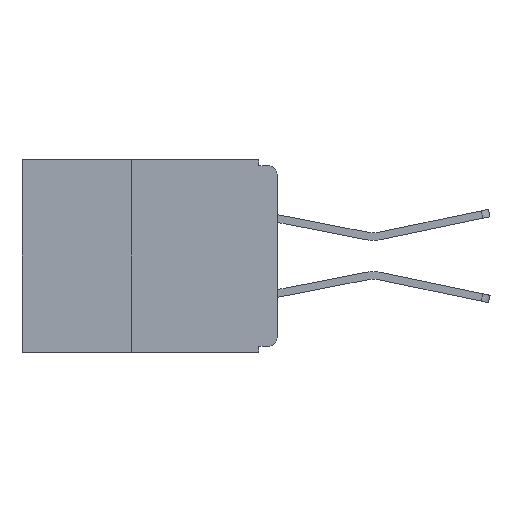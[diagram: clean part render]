
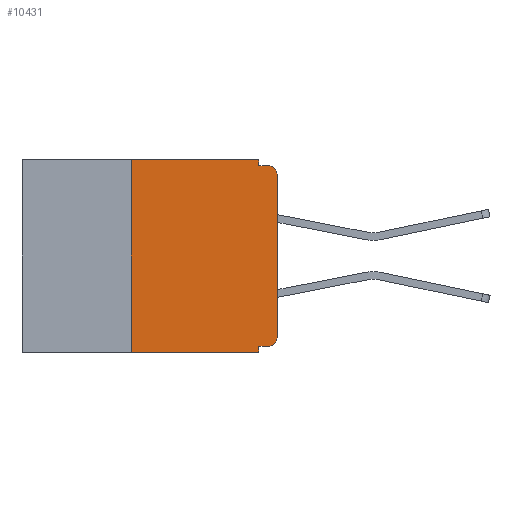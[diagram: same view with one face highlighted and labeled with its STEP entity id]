
A CAD part, left-side view. The second image highlights one B-rep face of the part: STEP entity #10431.
In plain terms, the highlighted planar face has unit normal (-1, 0, 0).
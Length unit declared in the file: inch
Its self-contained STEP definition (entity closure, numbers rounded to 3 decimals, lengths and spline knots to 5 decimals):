
#203 = CARTESIAN_POINT ( 'NONE',  ( 0., 0.031, 0. ) ) ;
#400 = CARTESIAN_POINT ( 'NONE',  ( 0., 0., -0.01 ) ) ;
#616 = ORIENTED_EDGE ( 'NONE', *, *, #10566, .F. ) ;
#731 = EDGE_CURVE ( 'NONE', #3363, #6437, #2843, .T. ) ;
#968 = CARTESIAN_POINT ( 'NONE',  ( 0., 0.015, -0.025 ) ) ;
#974 = LINE ( 'NONE', #12995, #9092 ) ;
#1455 = VERTEX_POINT ( 'NONE', #6132 ) ;
#1554 = VECTOR ( 'NONE', #11753, 39.37008 ) ;
#1560 = CARTESIAN_POINT ( 'NONE',  ( 0., 0.25, 0. ) ) ;
#1798 = ORIENTED_EDGE ( 'NONE', *, *, #11743, .F. ) ;
#1991 = PLANE ( 'NONE',  #2355 ) ;
#2018 = DIRECTION ( 'NONE',  ( 0., 0., -1. ) ) ;
#2137 = LINE ( 'NONE', #8072, #4761 ) ;
#2355 = AXIS2_PLACEMENT_3D ( 'NONE', #3112, #4258, #11383 ) ;
#2638 = AXIS2_PLACEMENT_3D ( 'NONE', #8622, #8341, #4077 ) ;
#2678 = ORIENTED_EDGE ( 'NONE', *, *, #10644, .F. ) ;
#2767 = DIRECTION ( 'NONE',  ( 0., 1., 0. ) ) ;
#2843 = CIRCLE ( 'NONE', #2638, 0.015 ) ;
#3112 = CARTESIAN_POINT ( 'NONE',  ( 0., 0.437, 0. ) ) ;
#3325 = CARTESIAN_POINT ( 'NONE',  ( 0., 0.031, -0.01 ) ) ;
#3348 = VERTEX_POINT ( 'NONE', #3325 ) ;
#3363 = VERTEX_POINT ( 'NONE', #12486 ) ;
#3395 = ORIENTED_EDGE ( 'NONE', *, *, #13267, .F. ) ;
#3677 = DIRECTION ( 'NONE',  ( 0., -1., 0. ) ) ;
#4077 = DIRECTION ( 'NONE',  ( 0., 0., -1. ) ) ;
#4258 = DIRECTION ( 'NONE',  ( 1., 0., 0. ) ) ;
#4278 = ORIENTED_EDGE ( 'NONE', *, *, #731, .T. ) ;
#4408 = DIRECTION ( 'NONE',  ( 0., -1., 0. ) ) ;
#4569 = VECTOR ( 'NONE', #11627, 39.37008 ) ;
#4761 = VECTOR ( 'NONE', #2767, 39.37008 ) ;
#4828 = LINE ( 'NONE', #10770, #1554 ) ;
#4979 = VECTOR ( 'NONE', #5648, 39.37008 ) ;
#5104 = CARTESIAN_POINT ( 'NONE',  ( 0., 0.25, -0.33 ) ) ;
#5451 = ORIENTED_EDGE ( 'NONE', *, *, #7136, .T. ) ;
#5579 = LINE ( 'NONE', #400, #7977 ) ;
#5647 = VECTOR ( 'NONE', #12519, 39.37008 ) ;
#5648 = DIRECTION ( 'NONE',  ( 0., 0., -1. ) ) ;
#5718 = ORIENTED_EDGE ( 'NONE', *, *, #7608, .T. ) ;
#5966 = EDGE_CURVE ( 'NONE', #3363, #12352, #2137, .T. ) ;
#6132 = CARTESIAN_POINT ( 'NONE',  ( 0., 0.015, -0.01 ) ) ;
#6177 = ORIENTED_EDGE ( 'NONE', *, *, #6625, .F. ) ;
#6437 = VERTEX_POINT ( 'NONE', #12530 ) ;
#6625 = EDGE_CURVE ( 'NONE', #3348, #1455, #5579, .T. ) ;
#6684 = VERTEX_POINT ( 'NONE', #11894 ) ;
#6759 = EDGE_CURVE ( 'NONE', #6437, #6684, #974, .T. ) ;
#6869 = EDGE_LOOP ( 'NONE', ( #11303, #5718, #6177, #2678, #1798, #616, #5451, #3395, #8450, #4278 ) ) ;
#7136 = EDGE_CURVE ( 'NONE', #8105, #8847, #12618, .T. ) ;
#7501 = CARTESIAN_POINT ( 'NONE',  ( 0., 0.437, 0. ) ) ;
#7569 = CARTESIAN_POINT ( 'NONE',  ( 0., 0.031, -0.33 ) ) ;
#7608 = EDGE_CURVE ( 'NONE', #6684, #1455, #9383, .T. ) ;
#7977 = VECTOR ( 'NONE', #3677, 39.37008 ) ;
#8022 = DIRECTION ( 'NONE',  ( 0., 0., 1. ) ) ;
#8072 = CARTESIAN_POINT ( 'NONE',  ( 0., 0., -0.32 ) ) ;
#8105 = VERTEX_POINT ( 'NONE', #5104 ) ;
#8341 = DIRECTION ( 'NONE',  ( -1., 0., 0. ) ) ;
#8357 = LINE ( 'NONE', #11554, #5647 ) ;
#8390 = DIRECTION ( 'NONE',  ( -1., 0., 0. ) ) ;
#8450 = ORIENTED_EDGE ( 'NONE', *, *, #5966, .F. ) ;
#8622 = CARTESIAN_POINT ( 'NONE',  ( 0., 0.015, -0.305 ) ) ;
#8847 = VERTEX_POINT ( 'NONE', #7569 ) ;
#9092 = VECTOR ( 'NONE', #8022, 39.37008 ) ;
#9383 = CIRCLE ( 'NONE', #10646, 0.015 ) ;
#9658 = VERTEX_POINT ( 'NONE', #1560 ) ;
#10431 = ADVANCED_FACE ( 'NONE', ( #12851 ), #1991, .F. ) ;
#10524 = LINE ( 'NONE', #7501, #12210 ) ;
#10566 = EDGE_CURVE ( 'NONE', #8105, #9658, #8357, .T. ) ;
#10641 = CARTESIAN_POINT ( 'NONE',  ( 0., 0.437, -0.33 ) ) ;
#10644 = EDGE_CURVE ( 'NONE', #11835, #3348, #12692, .T. ) ;
#10646 = AXIS2_PLACEMENT_3D ( 'NONE', #968, #8390, #2018 ) ;
#10770 = CARTESIAN_POINT ( 'NONE',  ( 0., 0.031, -0.33 ) ) ;
#11303 = ORIENTED_EDGE ( 'NONE', *, *, #6759, .T. ) ;
#11345 = CARTESIAN_POINT ( 'NONE',  ( 0., 0.031, -0.32 ) ) ;
#11383 = DIRECTION ( 'NONE',  ( 0., 0., -1. ) ) ;
#11554 = CARTESIAN_POINT ( 'NONE',  ( 0., 0.25, -0.33 ) ) ;
#11627 = DIRECTION ( 'NONE',  ( 0., -1., 0. ) ) ;
#11743 = EDGE_CURVE ( 'NONE', #9658, #11835, #10524, .T. ) ;
#11753 = DIRECTION ( 'NONE',  ( 0., 0., -1. ) ) ;
#11835 = VERTEX_POINT ( 'NONE', #203 ) ;
#11894 = CARTESIAN_POINT ( 'NONE',  ( 0., 0., -0.025 ) ) ;
#12210 = VECTOR ( 'NONE', #4408, 39.37008 ) ;
#12352 = VERTEX_POINT ( 'NONE', #11345 ) ;
#12486 = CARTESIAN_POINT ( 'NONE',  ( 0., 0.015, -0.32 ) ) ;
#12519 = DIRECTION ( 'NONE',  ( 0., 0., 1. ) ) ;
#12530 = CARTESIAN_POINT ( 'NONE',  ( 0., 0., -0.305 ) ) ;
#12618 = LINE ( 'NONE', #10641, #4569 ) ;
#12652 = CARTESIAN_POINT ( 'NONE',  ( 0., 0.031, 0. ) ) ;
#12692 = LINE ( 'NONE', #12652, #4979 ) ;
#12851 = FACE_OUTER_BOUND ( 'NONE', #6869, .T. ) ;
#12995 = CARTESIAN_POINT ( 'NONE',  ( 0., 0., 0. ) ) ;
#13267 = EDGE_CURVE ( 'NONE', #12352, #8847, #4828, .T. ) ;
